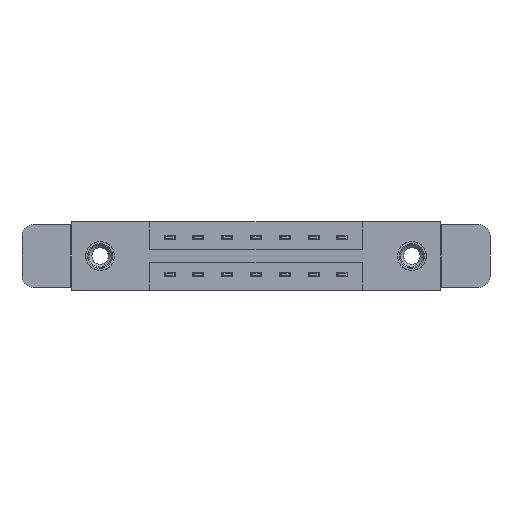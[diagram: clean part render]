
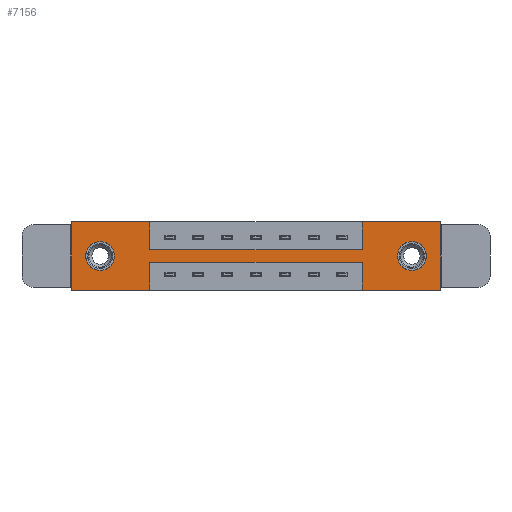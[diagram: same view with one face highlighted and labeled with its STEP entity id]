
A CAD part, front view. The second image highlights one B-rep face of the part: STEP entity #7156.
In plain terms, the highlighted planar face has unit normal (0, -1, 0).
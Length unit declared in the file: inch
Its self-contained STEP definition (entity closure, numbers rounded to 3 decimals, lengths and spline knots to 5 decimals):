
#16 = ORIENTED_EDGE ( 'NONE', *, *, #6678, .T. ) ;
#98 = EDGE_CURVE ( 'NONE', #7105, #161, #800, .T. ) ;
#147 = ORIENTED_EDGE ( 'NONE', *, *, #9783, .F. ) ;
#161 = VERTEX_POINT ( 'NONE', #2650 ) ;
#165 = VERTEX_POINT ( 'NONE', #12103 ) ;
#190 = EDGE_LOOP ( 'NONE', ( #7234, #940, #326, #2973, #1105, #147, #8702, #2926, #2761, #4563, #2024, #2110 ) ) ;
#326 = ORIENTED_EDGE ( 'NONE', *, *, #4306, .F. ) ;
#384 = VERTEX_POINT ( 'NONE', #1565 ) ;
#427 = DIRECTION ( 'NONE',  ( 0., 0., 1. ) ) ;
#464 = DIRECTION ( 'NONE',  ( -1., 0., 0. ) ) ;
#591 = FACE_OUTER_BOUND ( 'NONE', #190, .T. ) ;
#618 = LINE ( 'NONE', #1469, #12333 ) ;
#620 = CARTESIAN_POINT ( 'NONE',  ( 0.425, 0., -0.37 ) ) ;
#682 = CARTESIAN_POINT ( 'NONE',  ( 0., 0., 0. ) ) ;
#800 = LINE ( 'NONE', #11034, #2771 ) ;
#841 = LINE ( 'NONE', #682, #7912 ) ;
#940 = ORIENTED_EDGE ( 'NONE', *, *, #98, .F. ) ;
#1105 = ORIENTED_EDGE ( 'NONE', *, *, #4036, .F. ) ;
#1128 = CARTESIAN_POINT ( 'NONE',  ( 1.843, 0., -0.185 ) ) ;
#1167 = DIRECTION ( 'NONE',  ( 0., 1., 0. ) ) ;
#1373 = CARTESIAN_POINT ( 'NONE',  ( 0., 0., 0. ) ) ;
#1382 = CARTESIAN_POINT ( 'NONE',  ( 1.573, 0., -0.37 ) ) ;
#1469 = CARTESIAN_POINT ( 'NONE',  ( 0., 0., -0.37 ) ) ;
#1495 = AXIS2_PLACEMENT_3D ( 'NONE', #2096, #5101, #11803 ) ;
#1496 = DIRECTION ( 'NONE',  ( 1., 0., 0. ) ) ;
#1565 = CARTESIAN_POINT ( 'NONE',  ( 0.425, 0., -0.37 ) ) ;
#1598 = DIRECTION ( 'NONE',  ( 0., 0., -1. ) ) ;
#1956 = CARTESIAN_POINT ( 'NONE',  ( 0., 0., -0.37 ) ) ;
#1983 = EDGE_CURVE ( 'NONE', #4228, #8646, #5126, .T. ) ;
#2024 = ORIENTED_EDGE ( 'NONE', *, *, #12190, .F. ) ;
#2096 = CARTESIAN_POINT ( 'NONE',  ( 1.843, 0., -0.185 ) ) ;
#2110 = ORIENTED_EDGE ( 'NONE', *, *, #6149, .F. ) ;
#2203 = AXIS2_PLACEMENT_3D ( 'NONE', #9570, #7614, #7649 ) ;
#2256 = CARTESIAN_POINT ( 'NONE',  ( 1.843, 0., -0.263 ) ) ;
#2347 = CARTESIAN_POINT ( 'NONE',  ( 0.425, 0., -0.15 ) ) ;
#2582 = AXIS2_PLACEMENT_3D ( 'NONE', #1128, #1167, #6975 ) ;
#2650 = CARTESIAN_POINT ( 'NONE',  ( 0.425, 0., -0.22 ) ) ;
#2682 = CARTESIAN_POINT ( 'NONE',  ( 1.573, 0., -0.22 ) ) ;
#2761 = ORIENTED_EDGE ( 'NONE', *, *, #6786, .F. ) ;
#2771 = VECTOR ( 'NONE', #3428, 39.37008 ) ;
#2779 = VECTOR ( 'NONE', #6076, 39.37008 ) ;
#2841 = DIRECTION ( 'NONE',  ( 0., 0., -1. ) ) ;
#2874 = VECTOR ( 'NONE', #3148, 39.37008 ) ;
#2926 = ORIENTED_EDGE ( 'NONE', *, *, #11125, .F. ) ;
#2973 = ORIENTED_EDGE ( 'NONE', *, *, #4034, .F. ) ;
#3148 = DIRECTION ( 'NONE',  ( 0., 0., -1. ) ) ;
#3428 = DIRECTION ( 'NONE',  ( -1., 0., 0. ) ) ;
#3525 = LINE ( 'NONE', #5238, #5933 ) ;
#3603 = PLANE ( 'NONE',  #7775 ) ;
#4023 = CARTESIAN_POINT ( 'NONE',  ( 0.425, 0., 0. ) ) ;
#4034 = EDGE_CURVE ( 'NONE', #5301, #4902, #3525, .T. ) ;
#4036 = EDGE_CURVE ( 'NONE', #7800, #5301, #8622, .T. ) ;
#4041 = CARTESIAN_POINT ( 'NONE',  ( 0.425, 0., 0. ) ) ;
#4055 = FACE_BOUND ( 'NONE', #10230, .T. ) ;
#4208 = ORIENTED_EDGE ( 'NONE', *, *, #8859, .T. ) ;
#4228 = VERTEX_POINT ( 'NONE', #2256 ) ;
#4306 = EDGE_CURVE ( 'NONE', #4902, #7105, #8769, .T. ) ;
#4338 = DIRECTION ( 'NONE',  ( 0., 1., 0. ) ) ;
#4510 = VERTEX_POINT ( 'NONE', #10449 ) ;
#4563 = ORIENTED_EDGE ( 'NONE', *, *, #9298, .F. ) ;
#4633 = EDGE_LOOP ( 'NONE', ( #16, #9601 ) ) ;
#4649 = AXIS2_PLACEMENT_3D ( 'NONE', #8379, #4338, #11076 ) ;
#4714 = VECTOR ( 'NONE', #5352, 39.37008 ) ;
#4819 = CIRCLE ( 'NONE', #1495, 0.078 ) ;
#4902 = VERTEX_POINT ( 'NONE', #5857 ) ;
#5060 = CARTESIAN_POINT ( 'NONE',  ( 1.573, 0., 0. ) ) ;
#5101 = DIRECTION ( 'NONE',  ( 0., 1., 0. ) ) ;
#5126 = CIRCLE ( 'NONE', #2582, 0.078 ) ;
#5217 = VERTEX_POINT ( 'NONE', #4041 ) ;
#5238 = CARTESIAN_POINT ( 'NONE',  ( 0., 0., -0.37 ) ) ;
#5301 = VERTEX_POINT ( 'NONE', #8835 ) ;
#5352 = DIRECTION ( 'NONE',  ( 0., 0., -1. ) ) ;
#5365 = CARTESIAN_POINT ( 'NONE',  ( 0.155, 0., -0.263 ) ) ;
#5428 = CARTESIAN_POINT ( 'NONE',  ( 1.843, 0., -0.107 ) ) ;
#5554 = CARTESIAN_POINT ( 'NONE',  ( 1.998, 0., 0. ) ) ;
#5575 = LINE ( 'NONE', #4023, #2874 ) ;
#5768 = CARTESIAN_POINT ( 'NONE',  ( 0.155, 0., -0.107 ) ) ;
#5857 = CARTESIAN_POINT ( 'NONE',  ( 1.573, 0., -0.37 ) ) ;
#5933 = VECTOR ( 'NONE', #6190, 39.37008 ) ;
#6076 = DIRECTION ( 'NONE',  ( 1., 0., 0. ) ) ;
#6149 = EDGE_CURVE ( 'NONE', #384, #9948, #618, .T. ) ;
#6188 = LINE ( 'NONE', #620, #11136 ) ;
#6190 = DIRECTION ( 'NONE',  ( -1., 0., 0. ) ) ;
#6339 = EDGE_CURVE ( 'NONE', #161, #384, #6188, .T. ) ;
#6678 = EDGE_CURVE ( 'NONE', #8646, #4228, #4819, .T. ) ;
#6713 = CARTESIAN_POINT ( 'NONE',  ( 0., 0., 0. ) ) ;
#6786 = EDGE_CURVE ( 'NONE', #5217, #7914, #5575, .T. ) ;
#6829 = VECTOR ( 'NONE', #10019, 39.37008 ) ;
#6970 = CARTESIAN_POINT ( 'NONE',  ( 0.425, 0., -0.15 ) ) ;
#6975 = DIRECTION ( 'NONE',  ( 0., 0., -1. ) ) ;
#7105 = VERTEX_POINT ( 'NONE', #2682 ) ;
#7112 = VECTOR ( 'NONE', #8669, 39.37008 ) ;
#7156 = ADVANCED_FACE ( 'NONE', ( #8701, #4055, #591 ), #3603, .T. ) ;
#7234 = ORIENTED_EDGE ( 'NONE', *, *, #6339, .F. ) ;
#7274 = VECTOR ( 'NONE', #427, 39.37008 ) ;
#7614 = DIRECTION ( 'NONE',  ( 0., 1., 0. ) ) ;
#7649 = DIRECTION ( 'NONE',  ( 0., 0., 1. ) ) ;
#7775 = AXIS2_PLACEMENT_3D ( 'NONE', #10320, #12383, #2841 ) ;
#7800 = VERTEX_POINT ( 'NONE', #5554 ) ;
#7912 = VECTOR ( 'NONE', #9267, 39.37008 ) ;
#7914 = VERTEX_POINT ( 'NONE', #6970 ) ;
#7921 = VECTOR ( 'NONE', #1496, 39.37008 ) ;
#8019 = VERTEX_POINT ( 'NONE', #5365 ) ;
#8112 = CARTESIAN_POINT ( 'NONE',  ( 1.573, 0., 0. ) ) ;
#8379 = CARTESIAN_POINT ( 'NONE',  ( 0.155, 0., -0.185 ) ) ;
#8622 = LINE ( 'NONE', #11924, #4714 ) ;
#8646 = VERTEX_POINT ( 'NONE', #5428 ) ;
#8669 = DIRECTION ( 'NONE',  ( 0., 0., 1. ) ) ;
#8701 = FACE_BOUND ( 'NONE', #4633, .T. ) ;
#8702 = ORIENTED_EDGE ( 'NONE', *, *, #11173, .F. ) ;
#8769 = LINE ( 'NONE', #1382, #6829 ) ;
#8835 = CARTESIAN_POINT ( 'NONE',  ( 1.998, 0., -0.37 ) ) ;
#8859 = EDGE_CURVE ( 'NONE', #8019, #10718, #11389, .T. ) ;
#9267 = DIRECTION ( 'NONE',  ( 1., 0., 0. ) ) ;
#9298 = EDGE_CURVE ( 'NONE', #165, #5217, #12404, .T. ) ;
#9403 = EDGE_CURVE ( 'NONE', #10718, #8019, #11376, .T. ) ;
#9570 = CARTESIAN_POINT ( 'NONE',  ( 0.155, 0., -0.185 ) ) ;
#9601 = ORIENTED_EDGE ( 'NONE', *, *, #1983, .T. ) ;
#9783 = EDGE_CURVE ( 'NONE', #10085, #7800, #841, .T. ) ;
#9948 = VERTEX_POINT ( 'NONE', #1956 ) ;
#10019 = DIRECTION ( 'NONE',  ( 0., 0., 1. ) ) ;
#10085 = VERTEX_POINT ( 'NONE', #5060 ) ;
#10230 = EDGE_LOOP ( 'NONE', ( #11641, #4208 ) ) ;
#10320 = CARTESIAN_POINT ( 'NONE',  ( 0., 0., -0.37 ) ) ;
#10449 = CARTESIAN_POINT ( 'NONE',  ( 1.573, 0., -0.15 ) ) ;
#10718 = VERTEX_POINT ( 'NONE', #5768 ) ;
#11034 = CARTESIAN_POINT ( 'NONE',  ( 0.425, 0., -0.22 ) ) ;
#11076 = DIRECTION ( 'NONE',  ( 0., 0., 1. ) ) ;
#11125 = EDGE_CURVE ( 'NONE', #7914, #4510, #11625, .T. ) ;
#11136 = VECTOR ( 'NONE', #1598, 39.37008 ) ;
#11173 = EDGE_CURVE ( 'NONE', #4510, #10085, #11329, .T. ) ;
#11329 = LINE ( 'NONE', #8112, #7274 ) ;
#11376 = CIRCLE ( 'NONE', #4649, 0.078 ) ;
#11389 = CIRCLE ( 'NONE', #2203, 0.078 ) ;
#11625 = LINE ( 'NONE', #2347, #2779 ) ;
#11641 = ORIENTED_EDGE ( 'NONE', *, *, #9403, .T. ) ;
#11803 = DIRECTION ( 'NONE',  ( 0., 0., -1. ) ) ;
#11883 = LINE ( 'NONE', #6713, #7112 ) ;
#11924 = CARTESIAN_POINT ( 'NONE',  ( 1.998, 0., 0. ) ) ;
#12103 = CARTESIAN_POINT ( 'NONE',  ( 0., 0., 0. ) ) ;
#12190 = EDGE_CURVE ( 'NONE', #9948, #165, #11883, .T. ) ;
#12333 = VECTOR ( 'NONE', #464, 39.37008 ) ;
#12383 = DIRECTION ( 'NONE',  ( 0., -1., 0. ) ) ;
#12404 = LINE ( 'NONE', #1373, #7921 ) ;
